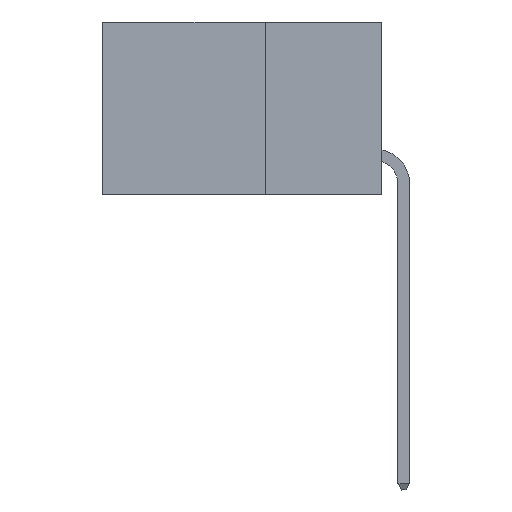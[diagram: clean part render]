
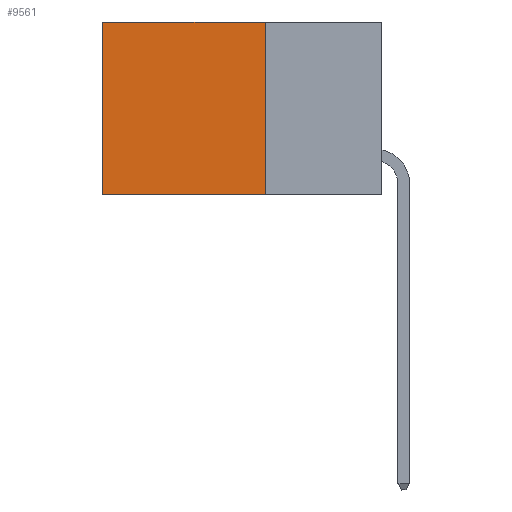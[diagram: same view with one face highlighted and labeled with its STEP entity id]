
A CAD part, left-side view. The second image highlights one B-rep face of the part: STEP entity #9561.
In plain terms, the highlighted planar face has unit normal (-1, 0, 0).
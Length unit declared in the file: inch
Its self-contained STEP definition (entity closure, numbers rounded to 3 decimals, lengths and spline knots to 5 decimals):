
#248 = CARTESIAN_POINT ( 'NONE',  ( 0.2875, 0.6, 0. ) ) ;
#697 = LINE ( 'NONE', #4189, #15783 ) ;
#753 = ORIENTED_EDGE ( 'NONE', *, *, #5725, .F. ) ;
#1509 = FACE_OUTER_BOUND ( 'NONE', #19575, .T. ) ;
#2396 = CARTESIAN_POINT ( 'NONE',  ( 0.2875, 0.25, -0.37 ) ) ;
#2525 = DIRECTION ( 'NONE',  ( 0., 1., 0. ) ) ;
#2645 = CARTESIAN_POINT ( 'NONE',  ( 0.2875, 0.25, 0. ) ) ;
#2996 = VERTEX_POINT ( 'NONE', #13543 ) ;
#4189 = CARTESIAN_POINT ( 'NONE',  ( 0.2875, 0.25, 0. ) ) ;
#4191 = ORIENTED_EDGE ( 'NONE', *, *, #7757, .T. ) ;
#4351 = EDGE_CURVE ( 'NONE', #2996, #16024, #697, .T. ) ;
#4392 = LINE ( 'NONE', #19379, #5943 ) ;
#4488 = LINE ( 'NONE', #2396, #16987 ) ;
#4847 = DIRECTION ( 'NONE',  ( 1., 0., 0. ) ) ;
#5446 = AXIS2_PLACEMENT_3D ( 'NONE', #19757, #4847, #14913 ) ;
#5603 = CARTESIAN_POINT ( 'NONE',  ( 0.2875, 0.6, -0.37 ) ) ;
#5725 = EDGE_CURVE ( 'NONE', #16024, #20868, #4488, .T. ) ;
#5943 = VECTOR ( 'NONE', #11459, 39.37008 ) ;
#7757 = EDGE_CURVE ( 'NONE', #13857, #20868, #4392, .T. ) ;
#9119 = DIRECTION ( 'NONE',  ( 0., 0., -1. ) ) ;
#9561 = ADVANCED_FACE ( 'NONE', ( #1509 ), #12301, .F. ) ;
#10555 = ORIENTED_EDGE ( 'NONE', *, *, #4351, .F. ) ;
#11384 = EDGE_CURVE ( 'NONE', #2996, #13857, #12230, .T. ) ;
#11459 = DIRECTION ( 'NONE',  ( 0., 0., -1. ) ) ;
#12230 = LINE ( 'NONE', #2645, #19365 ) ;
#12301 = PLANE ( 'NONE',  #5446 ) ;
#13419 = CARTESIAN_POINT ( 'NONE',  ( 0.2875, 0.25, -0.37 ) ) ;
#13543 = CARTESIAN_POINT ( 'NONE',  ( 0.2875, 0.25, 0. ) ) ;
#13857 = VERTEX_POINT ( 'NONE', #248 ) ;
#14913 = DIRECTION ( 'NONE',  ( 0., 0., -1. ) ) ;
#15294 = ORIENTED_EDGE ( 'NONE', *, *, #11384, .T. ) ;
#15783 = VECTOR ( 'NONE', #9119, 39.37008 ) ;
#16024 = VERTEX_POINT ( 'NONE', #13419 ) ;
#16987 = VECTOR ( 'NONE', #2525, 39.37008 ) ;
#19050 = DIRECTION ( 'NONE',  ( 0., 1., 0. ) ) ;
#19365 = VECTOR ( 'NONE', #19050, 39.37008 ) ;
#19379 = CARTESIAN_POINT ( 'NONE',  ( 0.2875, 0.6, 0. ) ) ;
#19575 = EDGE_LOOP ( 'NONE', ( #4191, #753, #10555, #15294 ) ) ;
#19757 = CARTESIAN_POINT ( 'NONE',  ( 0.2875, 0.25, 0. ) ) ;
#20868 = VERTEX_POINT ( 'NONE', #5603 ) ;
